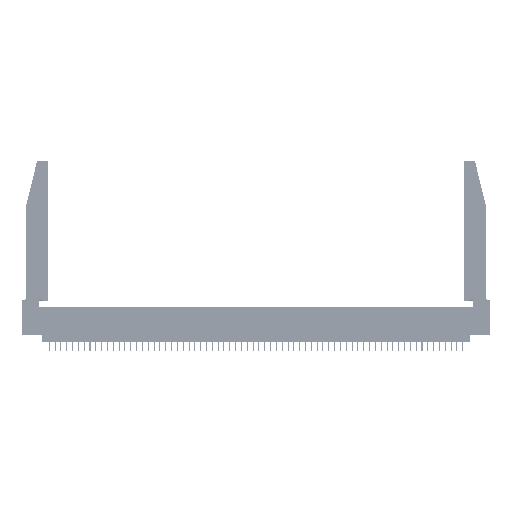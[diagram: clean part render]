
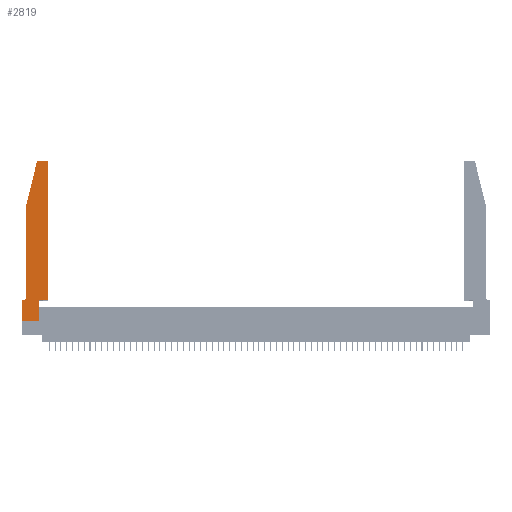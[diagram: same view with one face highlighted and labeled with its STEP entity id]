
A CAD part, top view. The second image highlights one B-rep face of the part: STEP entity #2819.
In plain terms, the highlighted planar face has unit normal (0, 0, 1).
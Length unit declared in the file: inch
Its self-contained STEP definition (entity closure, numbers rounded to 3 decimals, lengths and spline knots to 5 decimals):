
#47 = CARTESIAN_POINT ( 'NONE',  ( 0.4505, 2.72, 0.37 ) ) ;
#1434 = VERTEX_POINT ( 'NONE', #40733 ) ;
#1958 = EDGE_CURVE ( 'NONE', #1434, #33667, #14728, .T. ) ;
#2819 = ADVANCED_FACE ( 'NONE', ( #44936 ), #23445, .T. ) ;
#3793 = AXIS2_PLACEMENT_3D ( 'NONE', #19727, #10224, #28661 ) ;
#4469 = DIRECTION ( 'NONE',  ( 1., 0., 0. ) ) ;
#4796 = EDGE_CURVE ( 'NONE', #34186, #43204, #12749, .T. ) ;
#6431 = AXIS2_PLACEMENT_3D ( 'NONE', #48913, #48142, #4469 ) ;
#6642 = VERTEX_POINT ( 'NONE', #16411 ) ;
#7050 = ORIENTED_EDGE ( 'NONE', *, *, #44579, .T. ) ;
#8292 = ORIENTED_EDGE ( 'NONE', *, *, #52649, .T. ) ;
#8925 = LINE ( 'NONE', #21689, #28364 ) ;
#9432 = LINE ( 'NONE', #14559, #40684 ) ;
#10224 = DIRECTION ( 'NONE',  ( 0., 0., 1. ) ) ;
#11169 = CARTESIAN_POINT ( 'NONE',  ( 0.284, 2.75, 0.37 ) ) ;
#12155 = LINE ( 'NONE', #45321, #26114 ) ;
#12344 = VERTEX_POINT ( 'NONE', #11169 ) ;
#12749 = LINE ( 'NONE', #26770, #31516 ) ;
#14428 = DIRECTION ( 'NONE',  ( 0., -1., 0. ) ) ;
#14559 = CARTESIAN_POINT ( 'NONE',  ( 0.0755, 2., 0.37 ) ) ;
#14728 = LINE ( 'NONE', #39350, #19626 ) ;
#14761 = DIRECTION ( 'NONE',  ( -0.239, -0.971, 0. ) ) ;
#15186 = VERTEX_POINT ( 'NONE', #47 ) ;
#15264 = CARTESIAN_POINT ( 'NONE',  ( 0.2865, 0.35, 0.37 ) ) ;
#15752 = DIRECTION ( 'NONE',  ( 0., 1., 0. ) ) ;
#16128 = DIRECTION ( 'NONE',  ( 0., -1., 0. ) ) ;
#16411 = CARTESIAN_POINT ( 'NONE',  ( 0.0755, 0.42, 0.37 ) ) ;
#16619 = VERTEX_POINT ( 'NONE', #24318 ) ;
#18039 = ORIENTED_EDGE ( 'NONE', *, *, #1958, .T. ) ;
#18680 = CARTESIAN_POINT ( 'NONE',  ( 0.4505, 0.35, 0.37 ) ) ;
#18934 = DIRECTION ( 'NONE',  ( 1., 0., 0. ) ) ;
#19626 = VECTOR ( 'NONE', #35619, 39.37008 ) ;
#19727 = CARTESIAN_POINT ( 'NONE',  ( 0., 0.35, 0.37 ) ) ;
#19875 = EDGE_LOOP ( 'NONE', ( #53654, #48493, #34279, #8292, #23990, #32559, #35563, #18039, #21823, #27395, #7050, #54623 ) ) ;
#20773 = LINE ( 'NONE', #37870, #44391 ) ;
#21689 = CARTESIAN_POINT ( 'NONE',  ( 0.2605, 2.75, 0.37 ) ) ;
#21823 = ORIENTED_EDGE ( 'NONE', *, *, #42937, .T. ) ;
#23042 = DIRECTION ( 'NONE',  ( 0., 0., 1. ) ) ;
#23445 = PLANE ( 'NONE',  #3793 ) ;
#23990 = ORIENTED_EDGE ( 'NONE', *, *, #31773, .T. ) ;
#24318 = CARTESIAN_POINT ( 'NONE',  ( 0.25487, 2.72718, 0.37 ) ) ;
#24694 = CARTESIAN_POINT ( 'NONE',  ( 0., 0., 0.37 ) ) ;
#26114 = VECTOR ( 'NONE', #54267, 39.37008 ) ;
#26770 = CARTESIAN_POINT ( 'NONE',  ( 0.4505, 0.35, 0.37 ) ) ;
#27395 = ORIENTED_EDGE ( 'NONE', *, *, #4796, .T. ) ;
#28364 = VECTOR ( 'NONE', #35452, 39.37008 ) ;
#28661 = DIRECTION ( 'NONE',  ( 1., 0., 0. ) ) ;
#28673 = DIRECTION ( 'NONE',  ( 1., 0., 0. ) ) ;
#28980 = LINE ( 'NONE', #18680, #35210 ) ;
#29136 = LINE ( 'NONE', #24694, #49306 ) ;
#29553 = VERTEX_POINT ( 'NONE', #52817 ) ;
#29757 = CARTESIAN_POINT ( 'NONE',  ( 0.0055, 0.35, 0.37 ) ) ;
#30426 = EDGE_CURVE ( 'NONE', #16619, #50223, #9432, .T. ) ;
#30493 = CARTESIAN_POINT ( 'NONE',  ( 0.4505, 0.35, 0.37 ) ) ;
#30999 = CARTESIAN_POINT ( 'NONE',  ( 0.0755, 2., 0.37 ) ) ;
#31318 = AXIS2_PLACEMENT_3D ( 'NONE', #31389, #23042, #18934 ) ;
#31389 = CARTESIAN_POINT ( 'NONE',  ( 0.4205, 2.72, 0.37 ) ) ;
#31516 = VECTOR ( 'NONE', #28673, 39.37008 ) ;
#31773 = EDGE_CURVE ( 'NONE', #6642, #54742, #47557, .T. ) ;
#32559 = ORIENTED_EDGE ( 'NONE', *, *, #37949, .T. ) ;
#32919 = AXIS2_PLACEMENT_3D ( 'NONE', #38839, #42686, #47188 ) ;
#33667 = VERTEX_POINT ( 'NONE', #55718 ) ;
#34186 = VERTEX_POINT ( 'NONE', #15264 ) ;
#34279 = ORIENTED_EDGE ( 'NONE', *, *, #30426, .T. ) ;
#34531 = VECTOR ( 'NONE', #14428, 39.37008 ) ;
#35210 = VECTOR ( 'NONE', #40811, 39.37008 ) ;
#35452 = DIRECTION ( 'NONE',  ( -1., 0., 0. ) ) ;
#35563 = ORIENTED_EDGE ( 'NONE', *, *, #51256, .T. ) ;
#35619 = DIRECTION ( 'NONE',  ( 1., 0., 0. ) ) ;
#37870 = CARTESIAN_POINT ( 'NONE',  ( 0.2865, 0.35, 0.37 ) ) ;
#37949 = EDGE_CURVE ( 'NONE', #54742, #29553, #12155, .T. ) ;
#38839 = CARTESIAN_POINT ( 'NONE',  ( 0.0055, 0.42, 0.37 ) ) ;
#38891 = CIRCLE ( 'NONE', #6431, 0.03 ) ;
#39350 = CARTESIAN_POINT ( 'NONE',  ( 0., 0., 0.37 ) ) ;
#40395 = EDGE_CURVE ( 'NONE', #15186, #49403, #52994, .T. ) ;
#40684 = VECTOR ( 'NONE', #14761, 39.37008 ) ;
#40733 = CARTESIAN_POINT ( 'NONE',  ( 0., 0., 0.37 ) ) ;
#40811 = DIRECTION ( 'NONE',  ( 0., 1., 0. ) ) ;
#41481 = LINE ( 'NONE', #54427, #34531 ) ;
#42686 = DIRECTION ( 'NONE',  ( 0., 0., -1. ) ) ;
#42937 = EDGE_CURVE ( 'NONE', #33667, #34186, #20773, .T. ) ;
#43204 = VERTEX_POINT ( 'NONE', #30493 ) ;
#44391 = VECTOR ( 'NONE', #15752, 39.37008 ) ;
#44579 = EDGE_CURVE ( 'NONE', #43204, #15186, #28980, .T. ) ;
#44936 = FACE_OUTER_BOUND ( 'NONE', #19875, .T. ) ;
#45321 = CARTESIAN_POINT ( 'NONE',  ( 0.0755, 0.35, 0.37 ) ) ;
#47188 = DIRECTION ( 'NONE',  ( -1., 0., 0. ) ) ;
#47557 = CIRCLE ( 'NONE', #32919, 0.07 ) ;
#47772 = CARTESIAN_POINT ( 'NONE',  ( 0.4205, 2.75, 0.37 ) ) ;
#48142 = DIRECTION ( 'NONE',  ( 0., 0., 1. ) ) ;
#48493 = ORIENTED_EDGE ( 'NONE', *, *, #51457, .T. ) ;
#48913 = CARTESIAN_POINT ( 'NONE',  ( 0.284, 2.72, 0.37 ) ) ;
#49306 = VECTOR ( 'NONE', #16128, 39.37008 ) ;
#49403 = VERTEX_POINT ( 'NONE', #47772 ) ;
#50223 = VERTEX_POINT ( 'NONE', #30999 ) ;
#51256 = EDGE_CURVE ( 'NONE', #29553, #1434, #29136, .T. ) ;
#51457 = EDGE_CURVE ( 'NONE', #12344, #16619, #38891, .T. ) ;
#52095 = EDGE_CURVE ( 'NONE', #49403, #12344, #8925, .T. ) ;
#52649 = EDGE_CURVE ( 'NONE', #50223, #6642, #41481, .T. ) ;
#52817 = CARTESIAN_POINT ( 'NONE',  ( 0., 0.35, 0.37 ) ) ;
#52994 = CIRCLE ( 'NONE', #31318, 0.03 ) ;
#53654 = ORIENTED_EDGE ( 'NONE', *, *, #52095, .T. ) ;
#54267 = DIRECTION ( 'NONE',  ( -1., 0., 0. ) ) ;
#54427 = CARTESIAN_POINT ( 'NONE',  ( 0.0755, 2., 0.37 ) ) ;
#54623 = ORIENTED_EDGE ( 'NONE', *, *, #40395, .T. ) ;
#54742 = VERTEX_POINT ( 'NONE', #29757 ) ;
#55718 = CARTESIAN_POINT ( 'NONE',  ( 0.2865, 0., 0.37 ) ) ;
